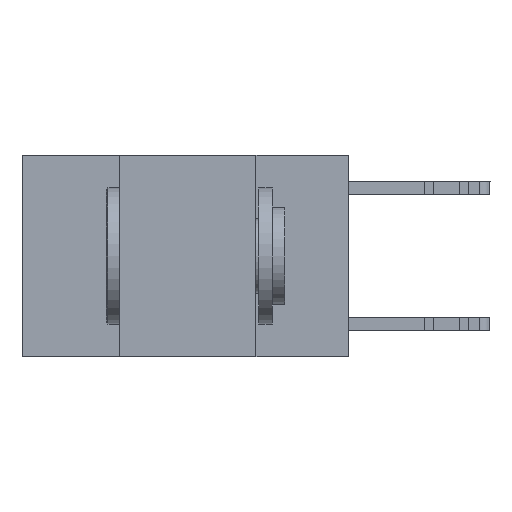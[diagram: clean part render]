
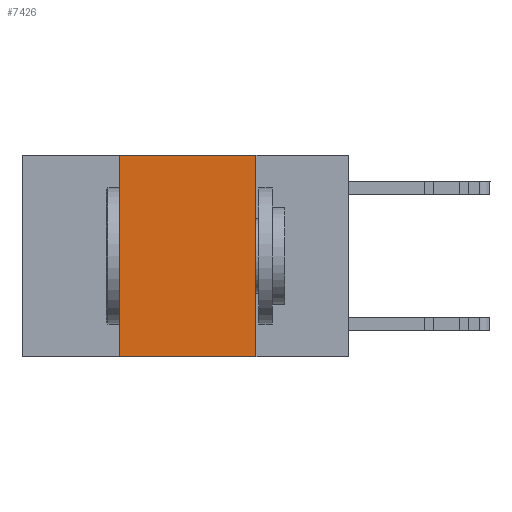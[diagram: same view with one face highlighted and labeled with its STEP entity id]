
A CAD part, left-side view. The second image highlights one B-rep face of the part: STEP entity #7426.
In plain terms, the highlighted planar face has unit normal (-1, 0, 0).
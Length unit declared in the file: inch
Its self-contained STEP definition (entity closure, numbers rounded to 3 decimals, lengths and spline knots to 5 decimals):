
#435 = VECTOR ( 'NONE', #30132, 39.37008 ) ;
#2775 = EDGE_CURVE ( 'NONE', #8339, #6435, #27482, .T. ) ;
#3845 = VECTOR ( 'NONE', #25312, 39.37008 ) ;
#6435 = VERTEX_POINT ( 'NONE', #21229 ) ;
#7389 = ORIENTED_EDGE ( 'NONE', *, *, #2775, .F. ) ;
#7426 = ADVANCED_FACE ( 'NONE', ( #24664 ), #17231, .F. ) ;
#7832 = CARTESIAN_POINT ( 'NONE',  ( 0., 0.17, 0. ) ) ;
#8339 = VERTEX_POINT ( 'NONE', #26469 ) ;
#9171 = CARTESIAN_POINT ( 'NONE',  ( 0., 0.17, 0. ) ) ;
#9234 = CARTESIAN_POINT ( 'NONE',  ( 0., 0.42, 0. ) ) ;
#14602 = CARTESIAN_POINT ( 'NONE',  ( 0., 0.17, -0.37 ) ) ;
#17231 = PLANE ( 'NONE',  #20221 ) ;
#18207 = CARTESIAN_POINT ( 'NONE',  ( 0., 0.6, -0.37 ) ) ;
#18633 = EDGE_CURVE ( 'NONE', #21186, #22978, #28051, .T. ) ;
#19857 = DIRECTION ( 'NONE',  ( 0., 0., -1. ) ) ;
#19896 = ORIENTED_EDGE ( 'NONE', *, *, #27334, .F. ) ;
#20188 = ORIENTED_EDGE ( 'NONE', *, *, #18633, .F. ) ;
#20221 = AXIS2_PLACEMENT_3D ( 'NONE', #26694, #27009, #19857 ) ;
#20642 = LINE ( 'NONE', #25770, #435 ) ;
#21186 = VERTEX_POINT ( 'NONE', #7832 ) ;
#21229 = CARTESIAN_POINT ( 'NONE',  ( 0., 0.42, 0. ) ) ;
#21342 = ORIENTED_EDGE ( 'NONE', *, *, #26943, .T. ) ;
#22978 = VERTEX_POINT ( 'NONE', #14602 ) ;
#24664 = FACE_OUTER_BOUND ( 'NONE', #27424, .T. ) ;
#25185 = VECTOR ( 'NONE', #27675, 39.37008 ) ;
#25312 = DIRECTION ( 'NONE',  ( 0., 0., 1. ) ) ;
#25646 = LINE ( 'NONE', #18207, #25185 ) ;
#25770 = CARTESIAN_POINT ( 'NONE',  ( 0., 0.6, 0. ) ) ;
#26469 = CARTESIAN_POINT ( 'NONE',  ( 0., 0.42, -0.37 ) ) ;
#26694 = CARTESIAN_POINT ( 'NONE',  ( 0., 0.6, 0. ) ) ;
#26943 = EDGE_CURVE ( 'NONE', #8339, #22978, #25646, .T. ) ;
#27009 = DIRECTION ( 'NONE',  ( 1., 0., 0. ) ) ;
#27034 = VECTOR ( 'NONE', #28363, 39.37008 ) ;
#27334 = EDGE_CURVE ( 'NONE', #6435, #21186, #20642, .T. ) ;
#27424 = EDGE_LOOP ( 'NONE', ( #20188, #19896, #7389, #21342 ) ) ;
#27482 = LINE ( 'NONE', #9234, #3845 ) ;
#27675 = DIRECTION ( 'NONE',  ( 0., -1., 0. ) ) ;
#28051 = LINE ( 'NONE', #9171, #27034 ) ;
#28363 = DIRECTION ( 'NONE',  ( 0., 0., -1. ) ) ;
#30132 = DIRECTION ( 'NONE',  ( 0., -1., 0. ) ) ;
